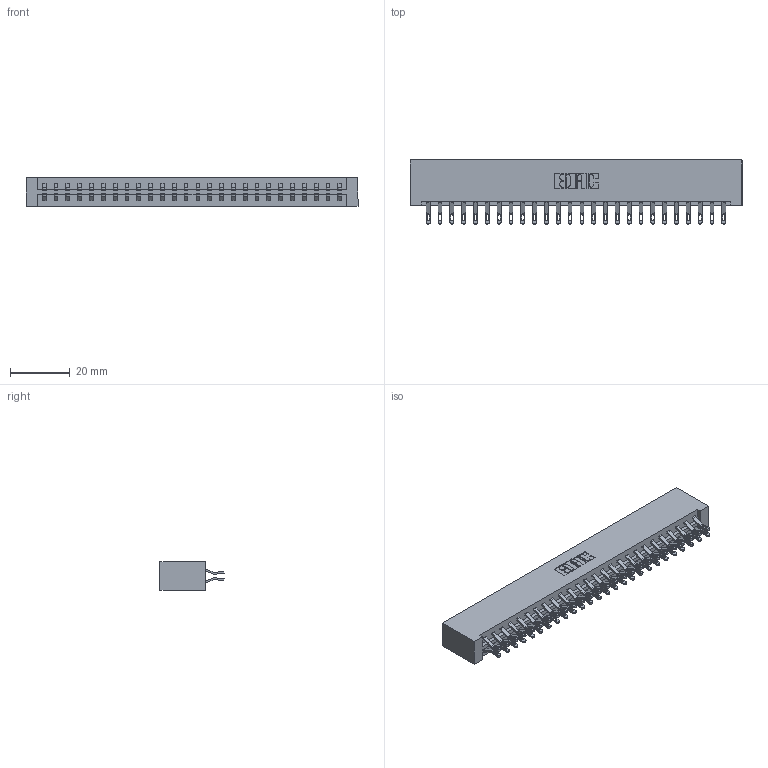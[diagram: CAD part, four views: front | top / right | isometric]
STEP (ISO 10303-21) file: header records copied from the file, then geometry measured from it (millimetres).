
FILE_DESCRIPTION (( 'STEP AP203' ), '1' );
FILE_NAME ('833-052-555-201.STEP', '2020-06-04T19:37:04', ( '' ), ( '' ), 'SwSTEP 2.0', 'SolidWorks 2020', '' );
FILE_SCHEMA (( 'CONFIG_CONTROL_DESIGN' ));
Length unit declared in the file: inch
Products named in the file (3): 345-292-001_555 Tail; 833-052-555-201; 833 Part_Lugless
Assembly tree (53 placements, depth 2):
  833-052-555-201
    833 Part_Lugless
    345-292-001_555 Tail  x52
Bounding box: 111.28 x 21.47 x 9.4 mm (x, y, z)
Volume: 11994.2 mm3; surface area: 14596.6 mm2
Topology: 53 solids, 53 shells, 3122 faces, 9803 edges, 6534 vertices
Faces by surface type: plane 1834, cylinder 1288
Entity records: 18845 total; most frequent: CARTESIAN_POINT 3176, ORIENTED_EDGE 3082, DIRECTION 2705, EDGE_CURVE 1541, VECTOR 1401, LINE 1401, VERTEX_POINT 1026, AXIS2_PLACEMENT_3D 652
